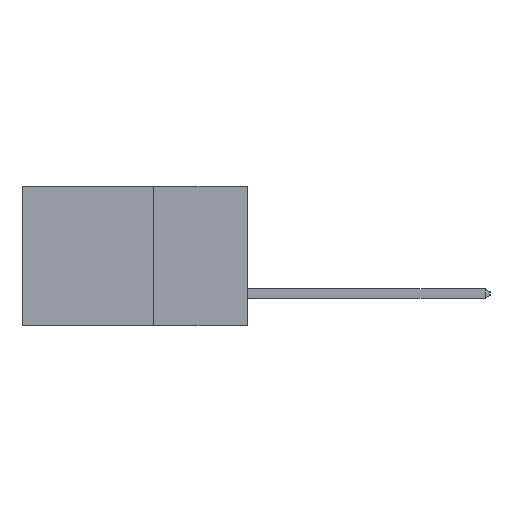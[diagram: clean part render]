
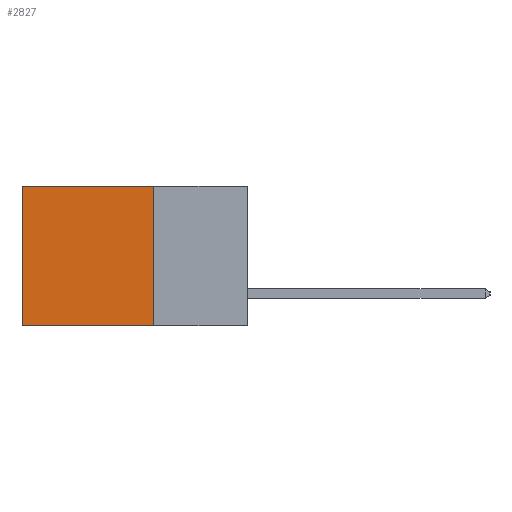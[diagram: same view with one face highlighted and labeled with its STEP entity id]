
A CAD part, left-side view. The second image highlights one B-rep face of the part: STEP entity #2827.
In plain terms, the highlighted planar face has unit normal (-1, 0, 0).
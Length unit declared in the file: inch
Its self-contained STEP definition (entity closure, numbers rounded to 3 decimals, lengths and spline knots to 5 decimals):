
#522 = CARTESIAN_POINT ( 'NONE',  ( 0.2615, 0.6, -0.37 ) ) ;
#1679 = FACE_OUTER_BOUND ( 'NONE', #11859, .T. ) ;
#1750 = DIRECTION ( 'NONE',  ( 0., 0., -1. ) ) ;
#1857 = CARTESIAN_POINT ( 'NONE',  ( 0.2615, 0.25, 0. ) ) ;
#2821 = AXIS2_PLACEMENT_3D ( 'NONE', #8153, #8107, #7978 ) ;
#2827 = ADVANCED_FACE ( 'NONE', ( #1679 ), #8419, .F. ) ;
#2834 = ORIENTED_EDGE ( 'NONE', *, *, #3125, .F. ) ;
#3125 = EDGE_CURVE ( 'NONE', #13016, #7512, #9901, .T. ) ;
#3799 = CARTESIAN_POINT ( 'NONE',  ( 0.2615, 0.6, -0.37 ) ) ;
#5086 = CARTESIAN_POINT ( 'NONE',  ( 0.2615, 0.25, -0.37 ) ) ;
#5197 = EDGE_CURVE ( 'NONE', #7512, #14529, #9639, .T. ) ;
#5529 = ORIENTED_EDGE ( 'NONE', *, *, #5197, .F. ) ;
#5541 = LINE ( 'NONE', #13721, #11338 ) ;
#6235 = VECTOR ( 'NONE', #8921, 39.37008 ) ;
#6888 = DIRECTION ( 'NONE',  ( 0., 1., 0. ) ) ;
#7364 = ORIENTED_EDGE ( 'NONE', *, *, #10487, .T. ) ;
#7512 = VERTEX_POINT ( 'NONE', #5086 ) ;
#7978 = DIRECTION ( 'NONE',  ( 0., 0., -1. ) ) ;
#8107 = DIRECTION ( 'NONE',  ( 1., 0., 0. ) ) ;
#8139 = CARTESIAN_POINT ( 'NONE',  ( 0.2615, 0.25, -0.37 ) ) ;
#8153 = CARTESIAN_POINT ( 'NONE',  ( 0.2615, 0.25, -0.37 ) ) ;
#8262 = ORIENTED_EDGE ( 'NONE', *, *, #14767, .T. ) ;
#8419 = PLANE ( 'NONE',  #2821 ) ;
#8921 = DIRECTION ( 'NONE',  ( 0., 0., -1. ) ) ;
#9639 = LINE ( 'NONE', #8139, #10034 ) ;
#9901 = LINE ( 'NONE', #14160, #6235 ) ;
#10034 = VECTOR ( 'NONE', #6888, 39.37008 ) ;
#10487 = EDGE_CURVE ( 'NONE', #13016, #11720, #5541, .T. ) ;
#11171 = VECTOR ( 'NONE', #1750, 39.37008 ) ;
#11338 = VECTOR ( 'NONE', #14898, 39.37008 ) ;
#11720 = VERTEX_POINT ( 'NONE', #15150 ) ;
#11859 = EDGE_LOOP ( 'NONE', ( #8262, #5529, #2834, #7364 ) ) ;
#13016 = VERTEX_POINT ( 'NONE', #1857 ) ;
#13721 = CARTESIAN_POINT ( 'NONE',  ( 0.2615, 0.25, 0. ) ) ;
#14160 = CARTESIAN_POINT ( 'NONE',  ( 0.2615, 0.25, -0.37 ) ) ;
#14529 = VERTEX_POINT ( 'NONE', #3799 ) ;
#14637 = LINE ( 'NONE', #522, #11171 ) ;
#14767 = EDGE_CURVE ( 'NONE', #11720, #14529, #14637, .T. ) ;
#14898 = DIRECTION ( 'NONE',  ( 0., 1., 0. ) ) ;
#15150 = CARTESIAN_POINT ( 'NONE',  ( 0.2615, 0.6, 0. ) ) ;
